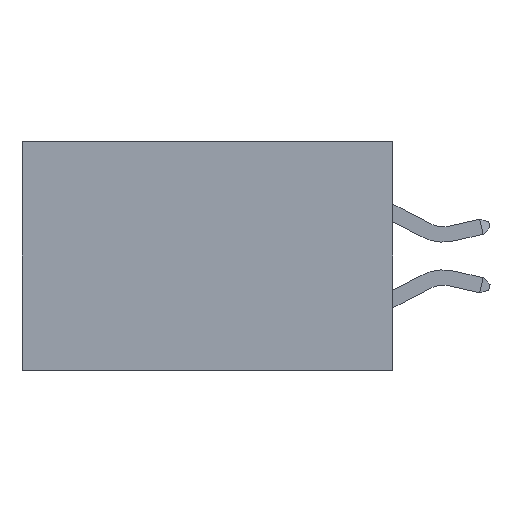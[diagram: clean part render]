
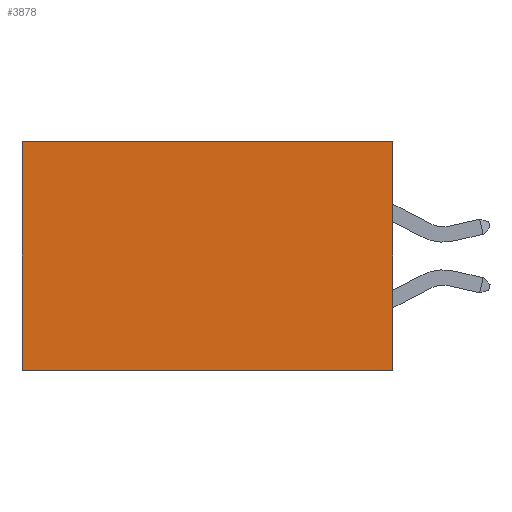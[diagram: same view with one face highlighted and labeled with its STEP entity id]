
A CAD part, left-side view. The second image highlights one B-rep face of the part: STEP entity #3878.
In plain terms, the highlighted planar face has unit normal (-1, 0, 0).
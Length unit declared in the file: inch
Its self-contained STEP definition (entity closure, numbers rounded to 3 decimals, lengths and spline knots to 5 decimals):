
#122 = DIRECTION ( 'NONE',  ( 0., 0., -1. ) ) ;
#752 = CARTESIAN_POINT ( 'NONE',  ( 0.2875, 0.6, -0.37 ) ) ;
#1128 = CARTESIAN_POINT ( 'NONE',  ( 0.2875, 0.6, 0. ) ) ;
#1185 = LINE ( 'NONE', #4107, #7039 ) ;
#1410 = CARTESIAN_POINT ( 'NONE',  ( 0.2875, 0., 0. ) ) ;
#1608 = EDGE_CURVE ( 'NONE', #6646, #6435, #4367, .T. ) ;
#1666 = ORIENTED_EDGE ( 'NONE', *, *, #5769, .T. ) ;
#2572 = VECTOR ( 'NONE', #7533, 39.37008 ) ;
#2736 = FACE_OUTER_BOUND ( 'NONE', #6100, .T. ) ;
#2751 = ORIENTED_EDGE ( 'NONE', *, *, #1608, .F. ) ;
#2801 = DIRECTION ( 'NONE',  ( 0., 0., -1. ) ) ;
#3794 = VECTOR ( 'NONE', #2801, 39.37008 ) ;
#3878 = ADVANCED_FACE ( 'NONE', ( #2736 ), #6930, .F. ) ;
#3879 = VERTEX_POINT ( 'NONE', #752 ) ;
#3951 = EDGE_CURVE ( 'NONE', #4143, #3879, #7860, .T. ) ;
#4107 = CARTESIAN_POINT ( 'NONE',  ( 0.2875, 0., 0. ) ) ;
#4143 = VERTEX_POINT ( 'NONE', #1128 ) ;
#4215 = ORIENTED_EDGE ( 'NONE', *, *, #3951, .T. ) ;
#4367 = LINE ( 'NONE', #1410, #2572 ) ;
#4841 = DIRECTION ( 'NONE',  ( 1., 0., 0. ) ) ;
#4972 = DIRECTION ( 'NONE',  ( 0., 1., 0. ) ) ;
#5397 = EDGE_CURVE ( 'NONE', #6435, #3879, #6833, .T. ) ;
#5425 = DIRECTION ( 'NONE',  ( 0., 1., 0. ) ) ;
#5769 = EDGE_CURVE ( 'NONE', #6646, #4143, #1185, .T. ) ;
#6100 = EDGE_LOOP ( 'NONE', ( #4215, #8235, #2751, #1666 ) ) ;
#6435 = VERTEX_POINT ( 'NONE', #6576 ) ;
#6576 = CARTESIAN_POINT ( 'NONE',  ( 0.2875, 0., -0.37 ) ) ;
#6646 = VERTEX_POINT ( 'NONE', #8271 ) ;
#6833 = LINE ( 'NONE', #7098, #8436 ) ;
#6930 = PLANE ( 'NONE',  #7837 ) ;
#7039 = VECTOR ( 'NONE', #5425, 39.37008 ) ;
#7098 = CARTESIAN_POINT ( 'NONE',  ( 0.2875, 0., -0.37 ) ) ;
#7533 = DIRECTION ( 'NONE',  ( 0., 0., -1. ) ) ;
#7592 = CARTESIAN_POINT ( 'NONE',  ( 0.2875, 0., 0. ) ) ;
#7837 = AXIS2_PLACEMENT_3D ( 'NONE', #7592, #4841, #122 ) ;
#7860 = LINE ( 'NONE', #8240, #3794 ) ;
#8235 = ORIENTED_EDGE ( 'NONE', *, *, #5397, .F. ) ;
#8240 = CARTESIAN_POINT ( 'NONE',  ( 0.2875, 0.6, 0. ) ) ;
#8271 = CARTESIAN_POINT ( 'NONE',  ( 0.2875, 0., 0. ) ) ;
#8436 = VECTOR ( 'NONE', #4972, 39.37008 ) ;
